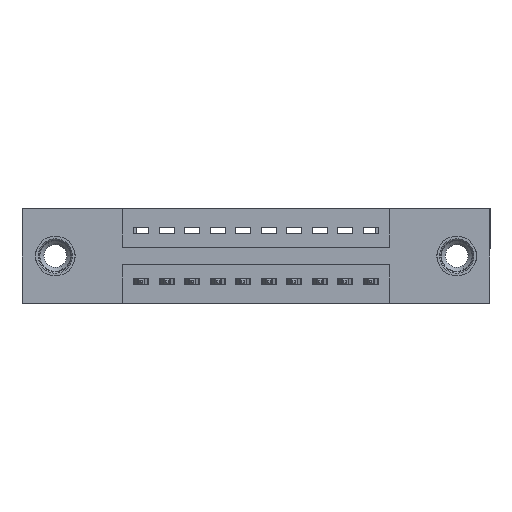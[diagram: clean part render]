
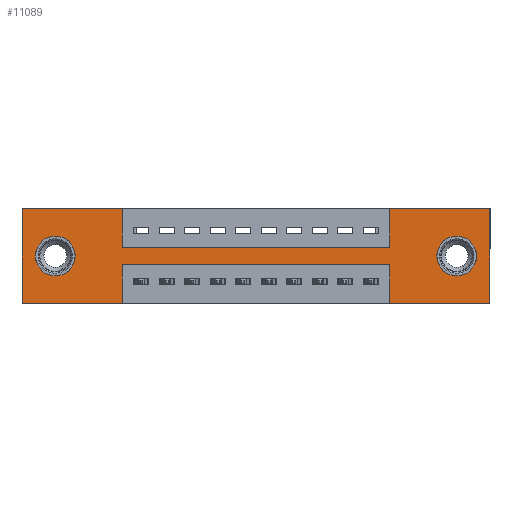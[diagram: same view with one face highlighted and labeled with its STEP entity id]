
A CAD part, front view. The second image highlights one B-rep face of the part: STEP entity #11089.
In plain terms, the highlighted planar face has unit normal (0, -1, 0).
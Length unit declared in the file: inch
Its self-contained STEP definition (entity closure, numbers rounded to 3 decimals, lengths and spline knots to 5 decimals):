
#73 = ORIENTED_EDGE ( 'NONE', *, *, #6808, .F. ) ;
#166 = LINE ( 'NONE', #15162, #14398 ) ;
#820 = CARTESIAN_POINT ( 'NONE',  ( 0., 0., 0. ) ) ;
#933 = EDGE_CURVE ( 'NONE', #5284, #12424, #1613, .T. ) ;
#1149 = ORIENTED_EDGE ( 'NONE', *, *, #8047, .F. ) ;
#1193 = CARTESIAN_POINT ( 'NONE',  ( 0., 0., 0. ) ) ;
#1243 = CARTESIAN_POINT ( 'NONE',  ( 0., 0., 0. ) ) ;
#1244 = CARTESIAN_POINT ( 'NONE',  ( 0.3925, 0., -0.37 ) ) ;
#1365 = CARTESIAN_POINT ( 'NONE',  ( 1.4425, 0., 0. ) ) ;
#1405 = EDGE_CURVE ( 'NONE', #2293, #8266, #12616, .T. ) ;
#1460 = ORIENTED_EDGE ( 'NONE', *, *, #14374, .F. ) ;
#1564 = VECTOR ( 'NONE', #11111, 39.37008 ) ;
#1597 = LINE ( 'NONE', #820, #13636 ) ;
#1603 = DIRECTION ( 'NONE',  ( 1., 0., 0. ) ) ;
#1613 = LINE ( 'NONE', #1243, #8171 ) ;
#1819 = EDGE_LOOP ( 'NONE', ( #11995, #14301 ) ) ;
#1850 = AXIS2_PLACEMENT_3D ( 'NONE', #7052, #10730, #12063 ) ;
#1907 = VERTEX_POINT ( 'NONE', #14201 ) ;
#2113 = AXIS2_PLACEMENT_3D ( 'NONE', #2226, #11599, #5219 ) ;
#2116 = VERTEX_POINT ( 'NONE', #8359 ) ;
#2226 = CARTESIAN_POINT ( 'NONE',  ( 1.705, 0., -0.185 ) ) ;
#2293 = VERTEX_POINT ( 'NONE', #11493 ) ;
#2359 = DIRECTION ( 'NONE',  ( 0., 1., 0. ) ) ;
#2497 = VERTEX_POINT ( 'NONE', #1193 ) ;
#2629 = LINE ( 'NONE', #8670, #10391 ) ;
#2827 = EDGE_LOOP ( 'NONE', ( #14425, #15615 ) ) ;
#3162 = CARTESIAN_POINT ( 'NONE',  ( 0.3925, 0., -0.22 ) ) ;
#3346 = AXIS2_PLACEMENT_3D ( 'NONE', #10859, #4327, #13178 ) ;
#3397 = CARTESIAN_POINT ( 'NONE',  ( 0.3925, 0., 0. ) ) ;
#3445 = AXIS2_PLACEMENT_3D ( 'NONE', #3850, #12819, #11442 ) ;
#3588 = CARTESIAN_POINT ( 'NONE',  ( 0.13, 0., -0.185 ) ) ;
#3799 = VERTEX_POINT ( 'NONE', #9225 ) ;
#3850 = CARTESIAN_POINT ( 'NONE',  ( 1.705, 0., -0.185 ) ) ;
#3975 = LINE ( 'NONE', #7251, #1564 ) ;
#4319 = EDGE_CURVE ( 'NONE', #1907, #2293, #16287, .T. ) ;
#4326 = ORIENTED_EDGE ( 'NONE', *, *, #8201, .F. ) ;
#4327 = DIRECTION ( 'NONE',  ( 0., -1., 0. ) ) ;
#4356 = CARTESIAN_POINT ( 'NONE',  ( 0., 0., -0.37 ) ) ;
#4608 = ORIENTED_EDGE ( 'NONE', *, *, #4319, .F. ) ;
#4774 = DIRECTION ( 'NONE',  ( 1., 0., 0. ) ) ;
#4777 = PLANE ( 'NONE',  #3346 ) ;
#4910 = DIRECTION ( 'NONE',  ( 0., 0., 1. ) ) ;
#4939 = DIRECTION ( 'NONE',  ( -1., 0., 0. ) ) ;
#5063 = FACE_OUTER_BOUND ( 'NONE', #8827, .T. ) ;
#5188 = CARTESIAN_POINT ( 'NONE',  ( 1.835, 0., -0.37 ) ) ;
#5208 = EDGE_CURVE ( 'NONE', #5483, #13602, #6412, .T. ) ;
#5219 = DIRECTION ( 'NONE',  ( 0., 0., -1. ) ) ;
#5284 = VERTEX_POINT ( 'NONE', #1365 ) ;
#5338 = CARTESIAN_POINT ( 'NONE',  ( 1.835, 0., 0. ) ) ;
#5483 = VERTEX_POINT ( 'NONE', #7862 ) ;
#6063 = CARTESIAN_POINT ( 'NONE',  ( 1.705, 0., -0.107 ) ) ;
#6118 = EDGE_CURVE ( 'NONE', #7843, #14017, #166, .T. ) ;
#6222 = VERTEX_POINT ( 'NONE', #10129 ) ;
#6347 = LINE ( 'NONE', #5338, #7710 ) ;
#6412 = CIRCLE ( 'NONE', #2113, 0.078 ) ;
#6444 = LINE ( 'NONE', #16456, #16303 ) ;
#6808 = EDGE_CURVE ( 'NONE', #12424, #7843, #6347, .T. ) ;
#7017 = VECTOR ( 'NONE', #15986, 39.37008 ) ;
#7052 = CARTESIAN_POINT ( 'NONE',  ( 0.13, 0., -0.185 ) ) ;
#7101 = CARTESIAN_POINT ( 'NONE',  ( 0.3925, 0., -0.15 ) ) ;
#7110 = VECTOR ( 'NONE', #10155, 39.37008 ) ;
#7185 = VECTOR ( 'NONE', #4774, 39.37008 ) ;
#7251 = CARTESIAN_POINT ( 'NONE',  ( 1.4425, 0., 0. ) ) ;
#7710 = VECTOR ( 'NONE', #14263, 39.37008 ) ;
#7843 = VERTEX_POINT ( 'NONE', #5188 ) ;
#7862 = CARTESIAN_POINT ( 'NONE',  ( 1.705, 0., -0.263 ) ) ;
#8012 = DIRECTION ( 'NONE',  ( -1., 0., 0. ) ) ;
#8047 = EDGE_CURVE ( 'NONE', #3799, #2116, #12961, .T. ) ;
#8171 = VECTOR ( 'NONE', #8973, 39.37008 ) ;
#8201 = EDGE_CURVE ( 'NONE', #16169, #3799, #16164, .T. ) ;
#8235 = ORIENTED_EDGE ( 'NONE', *, *, #6118, .F. ) ;
#8266 = VERTEX_POINT ( 'NONE', #8975 ) ;
#8359 = CARTESIAN_POINT ( 'NONE',  ( 0., 0., -0.37 ) ) ;
#8574 = CIRCLE ( 'NONE', #1850, 0.078 ) ;
#8670 = CARTESIAN_POINT ( 'NONE',  ( 0.3925, 0., -0.22 ) ) ;
#8827 = EDGE_LOOP ( 'NONE', ( #4326, #10442, #15362, #8235, #73, #14107, #1460, #16396, #4608, #10829, #14445, #1149 ) ) ;
#8973 = DIRECTION ( 'NONE',  ( 1., 0., 0. ) ) ;
#8975 = CARTESIAN_POINT ( 'NONE',  ( 1.4425, 0., -0.15 ) ) ;
#9225 = CARTESIAN_POINT ( 'NONE',  ( 0.3925, 0., -0.37 ) ) ;
#9945 = EDGE_CURVE ( 'NONE', #13602, #5483, #11082, .T. ) ;
#9964 = CARTESIAN_POINT ( 'NONE',  ( 1.835, 0., 0. ) ) ;
#10129 = CARTESIAN_POINT ( 'NONE',  ( 1.4425, 0., -0.22 ) ) ;
#10155 = DIRECTION ( 'NONE',  ( 0., 0., -1. ) ) ;
#10391 = VECTOR ( 'NONE', #4939, 39.37008 ) ;
#10442 = ORIENTED_EDGE ( 'NONE', *, *, #13432, .F. ) ;
#10730 = DIRECTION ( 'NONE',  ( 0., 1., 0. ) ) ;
#10759 = CARTESIAN_POINT ( 'NONE',  ( 1.4425, 0., -0.37 ) ) ;
#10829 = ORIENTED_EDGE ( 'NONE', *, *, #13507, .F. ) ;
#10859 = CARTESIAN_POINT ( 'NONE',  ( 0., 0., -0.37 ) ) ;
#10910 = VECTOR ( 'NONE', #8012, 39.37008 ) ;
#11002 = EDGE_CURVE ( 'NONE', #13543, #16574, #11893, .T. ) ;
#11082 = CIRCLE ( 'NONE', #3445, 0.078 ) ;
#11089 = ADVANCED_FACE ( 'NONE', ( #15312, #14926, #5063 ), #4777, .T. ) ;
#11111 = DIRECTION ( 'NONE',  ( 0., 0., 1. ) ) ;
#11442 = DIRECTION ( 'NONE',  ( 0., 0., -1. ) ) ;
#11493 = CARTESIAN_POINT ( 'NONE',  ( 0.3925, 0., -0.15 ) ) ;
#11599 = DIRECTION ( 'NONE',  ( 0., 1., 0. ) ) ;
#11893 = CIRCLE ( 'NONE', #14182, 0.078 ) ;
#11995 = ORIENTED_EDGE ( 'NONE', *, *, #13563, .T. ) ;
#12063 = DIRECTION ( 'NONE',  ( 0., 0., 1. ) ) ;
#12211 = EDGE_CURVE ( 'NONE', #14017, #6222, #6444, .T. ) ;
#12424 = VERTEX_POINT ( 'NONE', #9964 ) ;
#12616 = LINE ( 'NONE', #7101, #13843 ) ;
#12819 = DIRECTION ( 'NONE',  ( 0., 1., 0. ) ) ;
#12832 = LINE ( 'NONE', #14115, #7185 ) ;
#12961 = LINE ( 'NONE', #4356, #10910 ) ;
#13178 = DIRECTION ( 'NONE',  ( 0., 0., -1. ) ) ;
#13356 = CARTESIAN_POINT ( 'NONE',  ( 0.13, 0., -0.107 ) ) ;
#13432 = EDGE_CURVE ( 'NONE', #6222, #16169, #2629, .T. ) ;
#13507 = EDGE_CURVE ( 'NONE', #2497, #1907, #12832, .T. ) ;
#13543 = VERTEX_POINT ( 'NONE', #14409 ) ;
#13563 = EDGE_CURVE ( 'NONE', #16574, #13543, #8574, .T. ) ;
#13602 = VERTEX_POINT ( 'NONE', #6063 ) ;
#13617 = EDGE_CURVE ( 'NONE', #2116, #2497, #1597, .T. ) ;
#13636 = VECTOR ( 'NONE', #16288, 39.37008 ) ;
#13843 = VECTOR ( 'NONE', #1603, 39.37008 ) ;
#13896 = DIRECTION ( 'NONE',  ( 0., 0., 1. ) ) ;
#14017 = VERTEX_POINT ( 'NONE', #10759 ) ;
#14107 = ORIENTED_EDGE ( 'NONE', *, *, #933, .F. ) ;
#14115 = CARTESIAN_POINT ( 'NONE',  ( 0., 0., 0. ) ) ;
#14182 = AXIS2_PLACEMENT_3D ( 'NONE', #3588, #2359, #4910 ) ;
#14201 = CARTESIAN_POINT ( 'NONE',  ( 0.3925, 0., 0. ) ) ;
#14263 = DIRECTION ( 'NONE',  ( 0., 0., -1. ) ) ;
#14301 = ORIENTED_EDGE ( 'NONE', *, *, #11002, .T. ) ;
#14374 = EDGE_CURVE ( 'NONE', #8266, #5284, #3975, .T. ) ;
#14398 = VECTOR ( 'NONE', #16469, 39.37008 ) ;
#14409 = CARTESIAN_POINT ( 'NONE',  ( 0.13, 0., -0.263 ) ) ;
#14425 = ORIENTED_EDGE ( 'NONE', *, *, #9945, .T. ) ;
#14445 = ORIENTED_EDGE ( 'NONE', *, *, #13617, .F. ) ;
#14926 = FACE_BOUND ( 'NONE', #1819, .T. ) ;
#15162 = CARTESIAN_POINT ( 'NONE',  ( 0., 0., -0.37 ) ) ;
#15312 = FACE_BOUND ( 'NONE', #2827, .T. ) ;
#15362 = ORIENTED_EDGE ( 'NONE', *, *, #12211, .F. ) ;
#15615 = ORIENTED_EDGE ( 'NONE', *, *, #5208, .T. ) ;
#15986 = DIRECTION ( 'NONE',  ( 0., 0., -1. ) ) ;
#16164 = LINE ( 'NONE', #1244, #7110 ) ;
#16169 = VERTEX_POINT ( 'NONE', #3162 ) ;
#16287 = LINE ( 'NONE', #3397, #7017 ) ;
#16288 = DIRECTION ( 'NONE',  ( 0., 0., 1. ) ) ;
#16303 = VECTOR ( 'NONE', #13896, 39.37008 ) ;
#16396 = ORIENTED_EDGE ( 'NONE', *, *, #1405, .F. ) ;
#16456 = CARTESIAN_POINT ( 'NONE',  ( 1.4425, 0., -0.37 ) ) ;
#16469 = DIRECTION ( 'NONE',  ( -1., 0., 0. ) ) ;
#16574 = VERTEX_POINT ( 'NONE', #13356 ) ;
